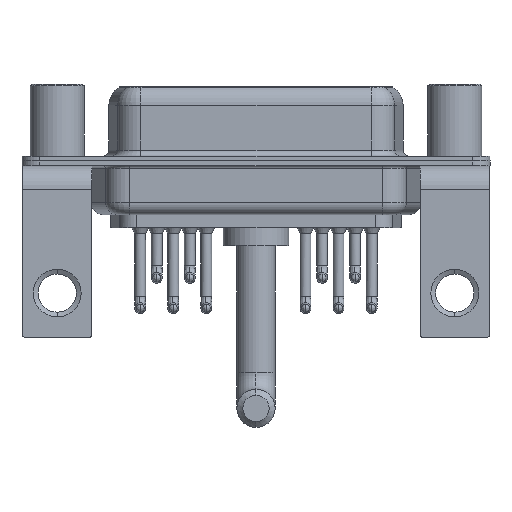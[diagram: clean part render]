
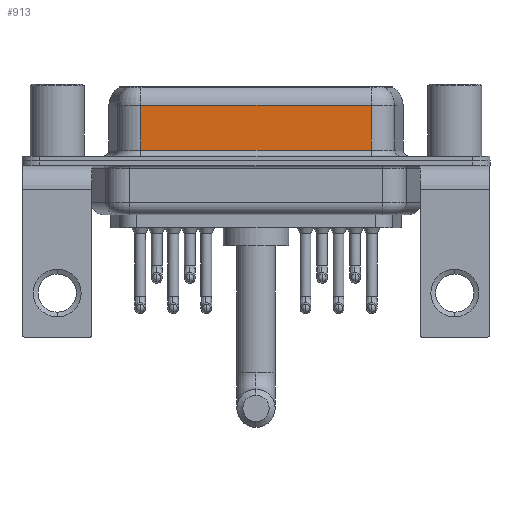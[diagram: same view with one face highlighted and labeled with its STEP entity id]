
A CAD part, front view. The second image highlights one B-rep face of the part: STEP entity #913.
In plain terms, the highlighted planar face has unit normal (0, -1, 0).
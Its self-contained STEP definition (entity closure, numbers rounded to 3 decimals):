
#99 = CARTESIAN_POINT ( 'NONE',  ( 26.287, -3.95, 4.65 ) ) ;
#913 = ADVANCED_FACE ( 'NONE', ( #20866 ), #9721, .F. ) ;
#1068 = CARTESIAN_POINT ( 'NONE',  ( 7.013, -3.95, 6.4 ) ) ;
#2036 = CARTESIAN_POINT ( 'NONE',  ( 7.013, -3.95, 0.9 ) ) ;
#3114 = LINE ( 'NONE', #9865, #6957 ) ;
#3533 = VERTEX_POINT ( 'NONE', #2036 ) ;
#4467 = DIRECTION ( 'NONE',  ( 0., 0., -1. ) ) ;
#4644 = ORIENTED_EDGE ( 'NONE', *, *, #5476, .T. ) ;
#5168 = EDGE_CURVE ( 'NONE', #11042, #3533, #14040, .T. ) ;
#5257 = EDGE_CURVE ( 'NONE', #16997, #11042, #6218, .T. ) ;
#5476 = EDGE_CURVE ( 'NONE', #3533, #12597, #3114, .T. ) ;
#5692 = DIRECTION ( 'NONE',  ( 0., 0., -1. ) ) ;
#6218 = LINE ( 'NONE', #99, #16838 ) ;
#6301 = EDGE_CURVE ( 'NONE', #16997, #12597, #11426, .T. ) ;
#6507 = DIRECTION ( 'NONE',  ( 0., 1., 0. ) ) ;
#6957 = VECTOR ( 'NONE', #11367, 1000. ) ;
#7141 = AXIS2_PLACEMENT_3D ( 'NONE', #14315, #6507, #14528 ) ;
#7634 = VECTOR ( 'NONE', #5692, 1000. ) ;
#9362 = VECTOR ( 'NONE', #4467, 1000. ) ;
#9721 = PLANE ( 'NONE',  #7141 ) ;
#9865 = CARTESIAN_POINT ( 'NONE',  ( 26.287, -3.95, 0.9 ) ) ;
#11042 = VERTEX_POINT ( 'NONE', #12010 ) ;
#11367 = DIRECTION ( 'NONE',  ( 1., 0., 0. ) ) ;
#11426 = LINE ( 'NONE', #14518, #9362 ) ;
#11468 = DIRECTION ( 'NONE',  ( -1., 0., 0. ) ) ;
#12010 = CARTESIAN_POINT ( 'NONE',  ( 7.013, -3.95, 4.65 ) ) ;
#12597 = VERTEX_POINT ( 'NONE', #16532 ) ;
#13327 = ORIENTED_EDGE ( 'NONE', *, *, #5257, .T. ) ;
#14040 = LINE ( 'NONE', #1068, #7634 ) ;
#14315 = CARTESIAN_POINT ( 'NONE',  ( 26.287, -3.95, 6.4 ) ) ;
#14518 = CARTESIAN_POINT ( 'NONE',  ( 26.287, -3.95, 6.4 ) ) ;
#14528 = DIRECTION ( 'NONE',  ( 0., 0., 1. ) ) ;
#14855 = ORIENTED_EDGE ( 'NONE', *, *, #6301, .F. ) ;
#15310 = EDGE_LOOP ( 'NONE', ( #14855, #13327, #16985, #4644 ) ) ;
#16347 = CARTESIAN_POINT ( 'NONE',  ( 26.287, -3.95, 4.65 ) ) ;
#16532 = CARTESIAN_POINT ( 'NONE',  ( 26.287, -3.95, 0.9 ) ) ;
#16838 = VECTOR ( 'NONE', #11468, 1000. ) ;
#16985 = ORIENTED_EDGE ( 'NONE', *, *, #5168, .T. ) ;
#16997 = VERTEX_POINT ( 'NONE', #16347 ) ;
#20866 = FACE_OUTER_BOUND ( 'NONE', #15310, .T. ) ;
